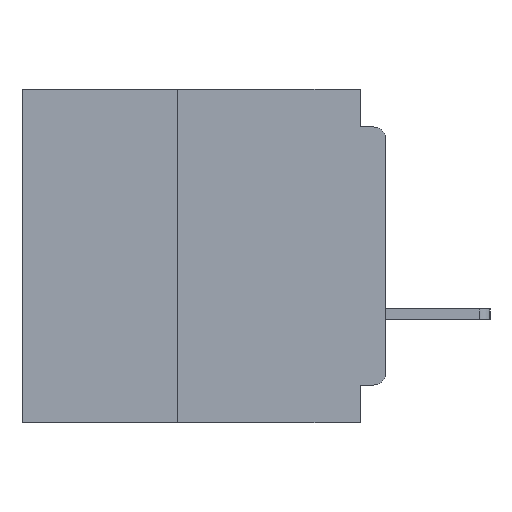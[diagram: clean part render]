
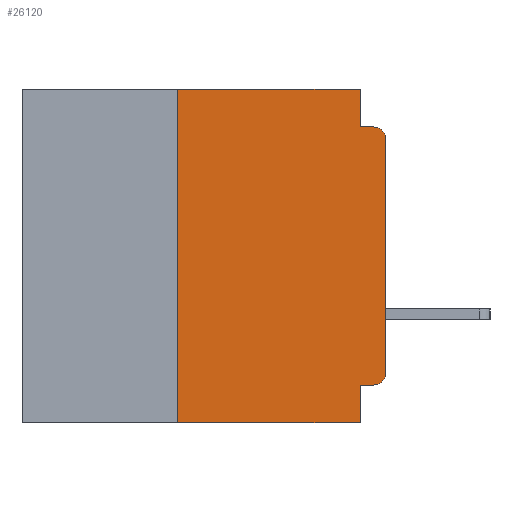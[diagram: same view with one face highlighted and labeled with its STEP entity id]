
A CAD part, left-side view. The second image highlights one B-rep face of the part: STEP entity #26120.
In plain terms, the highlighted planar face has unit normal (-1, 0, 0).
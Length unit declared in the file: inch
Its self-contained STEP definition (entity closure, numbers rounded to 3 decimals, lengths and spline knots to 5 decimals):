
#502 = EDGE_CURVE ( 'NONE', #25261, #5192, #16655, .T. ) ;
#1435 = AXIS2_PLACEMENT_3D ( 'NONE', #26988, #8370, #30076 ) ;
#1713 = ORIENTED_EDGE ( 'NONE', *, *, #22292, .T. ) ;
#1770 = CIRCLE ( 'NONE', #36697, 0.015 ) ;
#3014 = CARTESIAN_POINT ( 'NONE',  ( 0., 0., -0.34 ) ) ;
#3987 = EDGE_CURVE ( 'NONE', #19418, #9288, #37599, .T. ) ;
#4597 = CARTESIAN_POINT ( 'NONE',  ( 0., 0.031, 0. ) ) ;
#5015 = CARTESIAN_POINT ( 'NONE',  ( 0., 0., -0.045 ) ) ;
#5192 = VERTEX_POINT ( 'NONE', #10542 ) ;
#5710 = DIRECTION ( 'NONE',  ( 0., -1., 0. ) ) ;
#5966 = CARTESIAN_POINT ( 'NONE',  ( 0., 0.031, 0. ) ) ;
#6319 = CARTESIAN_POINT ( 'NONE',  ( 0., 0.25, -0.4 ) ) ;
#7049 = VECTOR ( 'NONE', #37389, 39.37008 ) ;
#7594 = ORIENTED_EDGE ( 'NONE', *, *, #33205, .F. ) ;
#7762 = ORIENTED_EDGE ( 'NONE', *, *, #11171, .F. ) ;
#8160 = DIRECTION ( 'NONE',  ( 0., -1., 0. ) ) ;
#8227 = VECTOR ( 'NONE', #5710, 39.37008 ) ;
#8299 = VECTOR ( 'NONE', #33775, 39.37008 ) ;
#8370 = DIRECTION ( 'NONE',  ( 1., 0., 0. ) ) ;
#8923 = ORIENTED_EDGE ( 'NONE', *, *, #502, .F. ) ;
#9288 = VERTEX_POINT ( 'NONE', #30145 ) ;
#9400 = DIRECTION ( 'NONE',  ( 0., 0., 1. ) ) ;
#10542 = CARTESIAN_POINT ( 'NONE',  ( 0., 0.031, -0.4 ) ) ;
#10979 = VECTOR ( 'NONE', #14369, 39.37008 ) ;
#11171 = EDGE_CURVE ( 'NONE', #9288, #31804, #23922, .T. ) ;
#11493 = CARTESIAN_POINT ( 'NONE',  ( 0., 0.031, -0.355 ) ) ;
#11714 = CARTESIAN_POINT ( 'NONE',  ( 0., 0.015, -0.045 ) ) ;
#11989 = LINE ( 'NONE', #23475, #10979 ) ;
#12306 = EDGE_CURVE ( 'NONE', #33667, #31804, #21520, .T. ) ;
#13248 = DIRECTION ( 'NONE',  ( -1., 0., 0. ) ) ;
#13291 = ORIENTED_EDGE ( 'NONE', *, *, #12306, .T. ) ;
#13974 = LINE ( 'NONE', #21061, #21183 ) ;
#14369 = DIRECTION ( 'NONE',  ( 0., -1., 0. ) ) ;
#14759 = CARTESIAN_POINT ( 'NONE',  ( 0., 0.015, -0.34 ) ) ;
#15136 = VERTEX_POINT ( 'NONE', #6319 ) ;
#15738 = ORIENTED_EDGE ( 'NONE', *, *, #38255, .F. ) ;
#15846 = CARTESIAN_POINT ( 'NONE',  ( 0., 0., 0. ) ) ;
#15986 = FACE_OUTER_BOUND ( 'NONE', #27649, .T. ) ;
#16076 = EDGE_CURVE ( 'NONE', #20011, #19418, #11989, .T. ) ;
#16592 = LINE ( 'NONE', #24852, #31072 ) ;
#16655 = LINE ( 'NONE', #24405, #8299 ) ;
#16940 = VERTEX_POINT ( 'NONE', #3014 ) ;
#17843 = DIRECTION ( 'NONE',  ( 0., 0., -1. ) ) ;
#18587 = VERTEX_POINT ( 'NONE', #26550 ) ;
#19228 = VECTOR ( 'NONE', #26366, 39.37008 ) ;
#19418 = VERTEX_POINT ( 'NONE', #5966 ) ;
#20011 = VERTEX_POINT ( 'NONE', #33260 ) ;
#20054 = EDGE_CURVE ( 'NONE', #15136, #5192, #30067, .T. ) ;
#21061 = CARTESIAN_POINT ( 'NONE',  ( 0., 0., -0.355 ) ) ;
#21183 = VECTOR ( 'NONE', #36456, 39.37008 ) ;
#21520 = CIRCLE ( 'NONE', #22042, 0.015 ) ;
#22042 = AXIS2_PLACEMENT_3D ( 'NONE', #31730, #13248, #34826 ) ;
#22292 = EDGE_CURVE ( 'NONE', #18587, #16940, #1770, .T. ) ;
#23475 = CARTESIAN_POINT ( 'NONE',  ( 0., 0.437, 0. ) ) ;
#23826 = PLANE ( 'NONE',  #1435 ) ;
#23922 = LINE ( 'NONE', #5015, #31223 ) ;
#24309 = CARTESIAN_POINT ( 'NONE',  ( 0., 0.437, -0.4 ) ) ;
#24405 = CARTESIAN_POINT ( 'NONE',  ( 0., 0.031, -0.4 ) ) ;
#24852 = CARTESIAN_POINT ( 'NONE',  ( 0., 0.25, -0.4 ) ) ;
#25261 = VERTEX_POINT ( 'NONE', #11493 ) ;
#26120 = ADVANCED_FACE ( 'NONE', ( #15986 ), #23826, .F. ) ;
#26366 = DIRECTION ( 'NONE',  ( 0., 0., -1. ) ) ;
#26550 = CARTESIAN_POINT ( 'NONE',  ( 0., 0.015, -0.355 ) ) ;
#26988 = CARTESIAN_POINT ( 'NONE',  ( 0., 0.437, 0. ) ) ;
#27649 = EDGE_LOOP ( 'NONE', ( #29383, #13291, #7762, #36167, #31289, #7594, #33549, #8923, #15738, #1713 ) ) ;
#29383 = ORIENTED_EDGE ( 'NONE', *, *, #38413, .T. ) ;
#30067 = LINE ( 'NONE', #24309, #8227 ) ;
#30076 = DIRECTION ( 'NONE',  ( 0., 0., -1. ) ) ;
#30145 = CARTESIAN_POINT ( 'NONE',  ( 0., 0.031, -0.045 ) ) ;
#30853 = LINE ( 'NONE', #15846, #7049 ) ;
#31072 = VECTOR ( 'NONE', #9400, 39.37008 ) ;
#31223 = VECTOR ( 'NONE', #8160, 39.37008 ) ;
#31289 = ORIENTED_EDGE ( 'NONE', *, *, #16076, .F. ) ;
#31730 = CARTESIAN_POINT ( 'NONE',  ( 0., 0.015, -0.06 ) ) ;
#31804 = VERTEX_POINT ( 'NONE', #11714 ) ;
#33205 = EDGE_CURVE ( 'NONE', #15136, #20011, #16592, .T. ) ;
#33260 = CARTESIAN_POINT ( 'NONE',  ( 0., 0.25, 0. ) ) ;
#33549 = ORIENTED_EDGE ( 'NONE', *, *, #20054, .T. ) ;
#33667 = VERTEX_POINT ( 'NONE', #39646 ) ;
#33775 = DIRECTION ( 'NONE',  ( 0., 0., -1. ) ) ;
#34826 = DIRECTION ( 'NONE',  ( 0., 0., -1. ) ) ;
#36167 = ORIENTED_EDGE ( 'NONE', *, *, #3987, .F. ) ;
#36323 = DIRECTION ( 'NONE',  ( -1., 0., 0. ) ) ;
#36456 = DIRECTION ( 'NONE',  ( 0., 1., 0. ) ) ;
#36697 = AXIS2_PLACEMENT_3D ( 'NONE', #14759, #36323, #17843 ) ;
#37389 = DIRECTION ( 'NONE',  ( 0., 0., 1. ) ) ;
#37599 = LINE ( 'NONE', #4597, #19228 ) ;
#38255 = EDGE_CURVE ( 'NONE', #18587, #25261, #13974, .T. ) ;
#38413 = EDGE_CURVE ( 'NONE', #16940, #33667, #30853, .T. ) ;
#39646 = CARTESIAN_POINT ( 'NONE',  ( 0., 0., -0.06 ) ) ;
